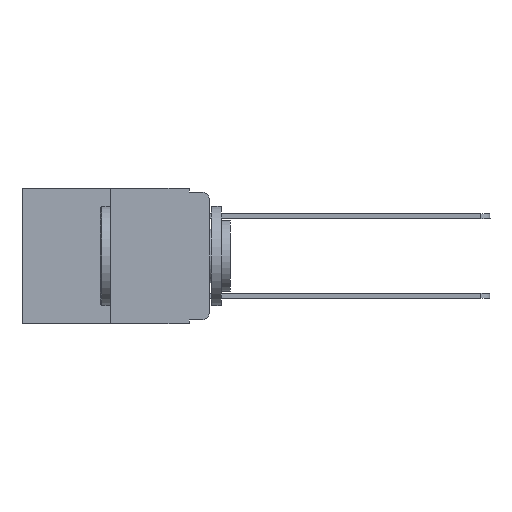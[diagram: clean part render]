
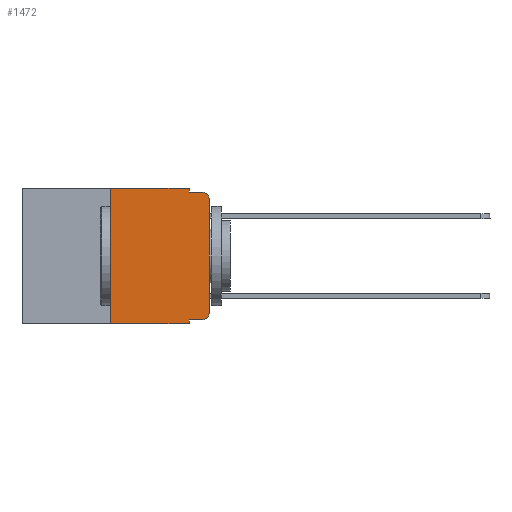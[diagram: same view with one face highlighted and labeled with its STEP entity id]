
A CAD part, left-side view. The second image highlights one B-rep face of the part: STEP entity #1472.
In plain terms, the highlighted planar face has unit normal (-1, 0, 0).
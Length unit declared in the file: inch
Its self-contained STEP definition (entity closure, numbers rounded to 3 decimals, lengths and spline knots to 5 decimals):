
#233 = CARTESIAN_POINT ( 'NONE',  ( 0., 0., 0. ) ) ;
#378 = LINE ( 'NONE', #5841, #2071 ) ;
#520 = EDGE_CURVE ( 'NONE', #8575, #10119, #4179, .T. ) ;
#567 = DIRECTION ( 'NONE',  ( 0., 0., -1. ) ) ;
#571 = CARTESIAN_POINT ( 'NONE',  ( 0., 0.25, 0. ) ) ;
#578 = VERTEX_POINT ( 'NONE', #5387 ) ;
#639 = CARTESIAN_POINT ( 'NONE',  ( 0., 0.473, 0. ) ) ;
#950 = CARTESIAN_POINT ( 'NONE',  ( 0., 0.02, -0.313 ) ) ;
#999 = CARTESIAN_POINT ( 'NONE',  ( 0., 0.051, 0. ) ) ;
#1090 = CARTESIAN_POINT ( 'NONE',  ( 0., 0.02, -0.01 ) ) ;
#1110 = EDGE_CURVE ( 'NONE', #578, #4611, #378, .T. ) ;
#1285 = CARTESIAN_POINT ( 'NONE',  ( 0., 0.051, -0.01 ) ) ;
#1394 = CIRCLE ( 'NONE', #2644, 0.02 ) ;
#1413 = VERTEX_POINT ( 'NONE', #5572 ) ;
#1472 = ADVANCED_FACE ( 'NONE', ( #5548 ), #4788, .F. ) ;
#1637 = EDGE_CURVE ( 'NONE', #4611, #9547, #1394, .T. ) ;
#1741 = CARTESIAN_POINT ( 'NONE',  ( 0., 0.25, -0.343 ) ) ;
#1746 = ORIENTED_EDGE ( 'NONE', *, *, #3896, .T. ) ;
#1904 = LINE ( 'NONE', #8003, #4888 ) ;
#1968 = VECTOR ( 'NONE', #6056, 39.37008 ) ;
#2071 = VECTOR ( 'NONE', #4253, 39.37008 ) ;
#2397 = CARTESIAN_POINT ( 'NONE',  ( 0., 0.473, 0. ) ) ;
#2469 = ORIENTED_EDGE ( 'NONE', *, *, #520, .F. ) ;
#2644 = AXIS2_PLACEMENT_3D ( 'NONE', #950, #7434, #8309 ) ;
#3055 = VERTEX_POINT ( 'NONE', #1741 ) ;
#3581 = CARTESIAN_POINT ( 'NONE',  ( 0., 0., -0.03 ) ) ;
#3792 = DIRECTION ( 'NONE',  ( 0., 0., 1. ) ) ;
#3896 = EDGE_CURVE ( 'NONE', #9547, #7893, #6145, .T. ) ;
#3948 = CARTESIAN_POINT ( 'NONE',  ( 0., 0.051, -0.01 ) ) ;
#4179 = LINE ( 'NONE', #10306, #1968 ) ;
#4253 = DIRECTION ( 'NONE',  ( 0., -1., 0. ) ) ;
#4390 = EDGE_CURVE ( 'NONE', #4412, #8575, #6146, .T. ) ;
#4412 = VERTEX_POINT ( 'NONE', #7385 ) ;
#4611 = VERTEX_POINT ( 'NONE', #5146 ) ;
#4717 = VERTEX_POINT ( 'NONE', #1090 ) ;
#4788 = PLANE ( 'NONE',  #4999 ) ;
#4888 = VECTOR ( 'NONE', #7185, 39.37008 ) ;
#4999 = AXIS2_PLACEMENT_3D ( 'NONE', #639, #6464, #567 ) ;
#5031 = CARTESIAN_POINT ( 'NONE',  ( 0., 0., -0.313 ) ) ;
#5146 = CARTESIAN_POINT ( 'NONE',  ( 0., 0.02, -0.333 ) ) ;
#5387 = CARTESIAN_POINT ( 'NONE',  ( 0., 0.051, -0.333 ) ) ;
#5513 = ORIENTED_EDGE ( 'NONE', *, *, #8960, .F. ) ;
#5548 = FACE_OUTER_BOUND ( 'NONE', #9555, .T. ) ;
#5572 = CARTESIAN_POINT ( 'NONE',  ( 0., 0.051, -0.343 ) ) ;
#5687 = ORIENTED_EDGE ( 'NONE', *, *, #1110, .T. ) ;
#5841 = CARTESIAN_POINT ( 'NONE',  ( 0., 0.051, -0.333 ) ) ;
#5872 = VECTOR ( 'NONE', #3792, 39.37008 ) ;
#6056 = DIRECTION ( 'NONE',  ( 0., 0., -1. ) ) ;
#6145 = LINE ( 'NONE', #233, #5872 ) ;
#6146 = LINE ( 'NONE', #2397, #7310 ) ;
#6270 = DIRECTION ( 'NONE',  ( 0., -1., 0. ) ) ;
#6327 = CIRCLE ( 'NONE', #7698, 0.02 ) ;
#6431 = DIRECTION ( 'NONE',  ( -1., 0., 0. ) ) ;
#6464 = DIRECTION ( 'NONE',  ( 1., 0., 0. ) ) ;
#6513 = ORIENTED_EDGE ( 'NONE', *, *, #9399, .T. ) ;
#7185 = DIRECTION ( 'NONE',  ( 0., -1., 0. ) ) ;
#7232 = LINE ( 'NONE', #571, #10003 ) ;
#7310 = VECTOR ( 'NONE', #9067, 39.37008 ) ;
#7348 = CARTESIAN_POINT ( 'NONE',  ( 0., 0.051, 0. ) ) ;
#7385 = CARTESIAN_POINT ( 'NONE',  ( 0., 0.25, 0. ) ) ;
#7434 = DIRECTION ( 'NONE',  ( -1., 0., 0. ) ) ;
#7698 = AXIS2_PLACEMENT_3D ( 'NONE', #9867, #6431, #10585 ) ;
#7741 = ORIENTED_EDGE ( 'NONE', *, *, #8116, .F. ) ;
#7893 = VERTEX_POINT ( 'NONE', #3581 ) ;
#8003 = CARTESIAN_POINT ( 'NONE',  ( 0., 0.473, -0.343 ) ) ;
#8042 = DIRECTION ( 'NONE',  ( 0., 0., 1. ) ) ;
#8116 = EDGE_CURVE ( 'NONE', #10119, #4717, #9491, .T. ) ;
#8305 = LINE ( 'NONE', #7348, #8564 ) ;
#8309 = DIRECTION ( 'NONE',  ( 0., 0., -1. ) ) ;
#8564 = VECTOR ( 'NONE', #10548, 39.37008 ) ;
#8575 = VERTEX_POINT ( 'NONE', #999 ) ;
#8711 = ORIENTED_EDGE ( 'NONE', *, *, #1637, .T. ) ;
#8881 = EDGE_CURVE ( 'NONE', #7893, #4717, #6327, .T. ) ;
#8960 = EDGE_CURVE ( 'NONE', #578, #1413, #8305, .T. ) ;
#8976 = EDGE_CURVE ( 'NONE', #3055, #4412, #7232, .T. ) ;
#9067 = DIRECTION ( 'NONE',  ( 0., -1., 0. ) ) ;
#9399 = EDGE_CURVE ( 'NONE', #3055, #1413, #1904, .T. ) ;
#9491 = LINE ( 'NONE', #1285, #10543 ) ;
#9547 = VERTEX_POINT ( 'NONE', #5031 ) ;
#9555 = EDGE_LOOP ( 'NONE', ( #1746, #10783, #7741, #2469, #10793, #10485, #6513, #5513, #5687, #8711 ) ) ;
#9867 = CARTESIAN_POINT ( 'NONE',  ( 0., 0.02, -0.03 ) ) ;
#10003 = VECTOR ( 'NONE', #8042, 39.37008 ) ;
#10119 = VERTEX_POINT ( 'NONE', #3948 ) ;
#10306 = CARTESIAN_POINT ( 'NONE',  ( 0., 0.051, 0. ) ) ;
#10485 = ORIENTED_EDGE ( 'NONE', *, *, #8976, .F. ) ;
#10543 = VECTOR ( 'NONE', #6270, 39.37008 ) ;
#10548 = DIRECTION ( 'NONE',  ( 0., 0., -1. ) ) ;
#10585 = DIRECTION ( 'NONE',  ( 0., 0., -1. ) ) ;
#10783 = ORIENTED_EDGE ( 'NONE', *, *, #8881, .T. ) ;
#10793 = ORIENTED_EDGE ( 'NONE', *, *, #4390, .F. ) ;
